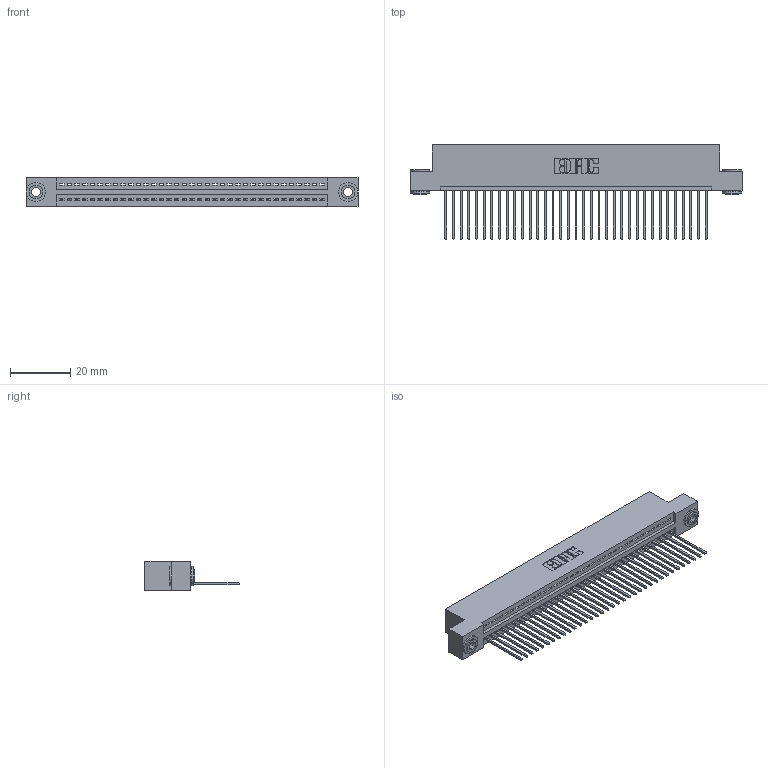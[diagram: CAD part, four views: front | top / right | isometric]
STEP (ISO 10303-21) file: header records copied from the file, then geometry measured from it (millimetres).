
FILE_DESCRIPTION (( 'STEP AP203' ), '1' );
FILE_NAME ('395-035-542-103.STEP', '2018-11-13T16:34:47', ( '' ), ( '' ), 'SwSTEP 2.0', 'SolidWorks 2016', '' );
FILE_SCHEMA (( 'CONFIG_CONTROL_DESIGN' ));
Length unit declared in the file: inch
Products named in the file (4): 345 Part_Flush Mounting Lugs - 0.156 Dia-TH; 345-250-002_345-250-002-102; 395-035-542-103; 345-292-001_345-293-142
Assembly tree (38 placements, depth 2):
  395-035-542-103
    345 Part_Flush Mounting Lugs - 0.156 Dia-TH
    345-292-001_345-293-142  x35
    345-250-002_345-250-002-102  x2
Bounding box: 110.11 x 31.29 x 9.4 mm (x, y, z)
Volume: 10498.2 mm3; surface area: 14563 mm2
Topology: 38 solids, 38 shells, 2194 faces, 6577 edges, 4334 vertices
Faces by surface type: plane 1490, cylinder 696, cone 8
Entity records: 27952 total; most frequent: CARTESIAN_POINT 4820, ORIENTED_EDGE 4782, DIRECTION 4251, EDGE_CURVE 2391, LINE 2095, VECTOR 2095, VERTEX_POINT 1590, AXIS2_PLACEMENT_3D 1078
